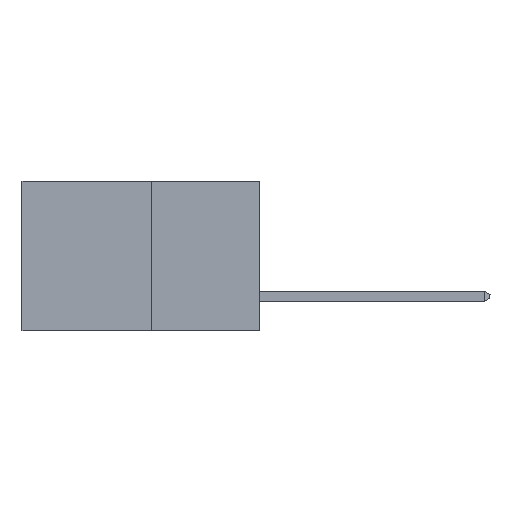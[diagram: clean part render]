
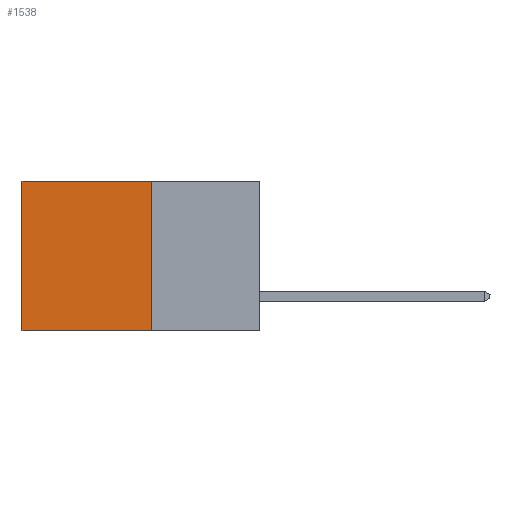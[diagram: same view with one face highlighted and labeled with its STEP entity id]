
A CAD part, left-side view. The second image highlights one B-rep face of the part: STEP entity #1538.
In plain terms, the highlighted planar face has unit normal (-1, 0, 0).
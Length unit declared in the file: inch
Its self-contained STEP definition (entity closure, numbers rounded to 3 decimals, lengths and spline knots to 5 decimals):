
#410 = CARTESIAN_POINT ( 'NONE',  ( 0.277, 0.59, -0.37 ) ) ;
#525 = LINE ( 'NONE', #6794, #6401 ) ;
#628 = CARTESIAN_POINT ( 'NONE',  ( 0.277, 0.27, -0.37 ) ) ;
#763 = CARTESIAN_POINT ( 'NONE',  ( 0.277, 0.27, -0.37 ) ) ;
#1269 = CARTESIAN_POINT ( 'NONE',  ( 0.277, 0.59, 0. ) ) ;
#1388 = DIRECTION ( 'NONE',  ( 1., 0., 0. ) ) ;
#1538 = ADVANCED_FACE ( 'NONE', ( #3960 ), #8419, .F. ) ;
#1837 = VERTEX_POINT ( 'NONE', #410 ) ;
#1838 = DIRECTION ( 'NONE',  ( 0., 1., 0. ) ) ;
#2000 = CARTESIAN_POINT ( 'NONE',  ( 0.277, 0.27, 0. ) ) ;
#2332 = VECTOR ( 'NONE', #1838, 39.37008 ) ;
#2643 = DIRECTION ( 'NONE',  ( 0., 0., -1. ) ) ;
#2728 = EDGE_CURVE ( 'NONE', #9635, #4302, #5594, .T. ) ;
#2854 = EDGE_CURVE ( 'NONE', #9635, #7333, #525, .T. ) ;
#3296 = DIRECTION ( 'NONE',  ( 0., 0., -1. ) ) ;
#3356 = ORIENTED_EDGE ( 'NONE', *, *, #2854, .T. ) ;
#3508 = LINE ( 'NONE', #7505, #7447 ) ;
#3830 = DIRECTION ( 'NONE',  ( 0., 0., -1. ) ) ;
#3960 = FACE_OUTER_BOUND ( 'NONE', #5766, .T. ) ;
#4297 = VECTOR ( 'NONE', #3296, 39.37008 ) ;
#4302 = VERTEX_POINT ( 'NONE', #763 ) ;
#4344 = DIRECTION ( 'NONE',  ( 0., 1., 0. ) ) ;
#4698 = EDGE_CURVE ( 'NONE', #4302, #1837, #6121, .T. ) ;
#5132 = ORIENTED_EDGE ( 'NONE', *, *, #4698, .F. ) ;
#5233 = AXIS2_PLACEMENT_3D ( 'NONE', #628, #1388, #2643 ) ;
#5374 = ORIENTED_EDGE ( 'NONE', *, *, #2728, .F. ) ;
#5594 = LINE ( 'NONE', #8568, #4297 ) ;
#5718 = CARTESIAN_POINT ( 'NONE',  ( 0.277, 0.27, -0.37 ) ) ;
#5766 = EDGE_LOOP ( 'NONE', ( #7102, #5132, #5374, #3356 ) ) ;
#6121 = LINE ( 'NONE', #5718, #2332 ) ;
#6401 = VECTOR ( 'NONE', #4344, 39.37008 ) ;
#6794 = CARTESIAN_POINT ( 'NONE',  ( 0.277, 0.27, 0. ) ) ;
#7102 = ORIENTED_EDGE ( 'NONE', *, *, #9208, .T. ) ;
#7333 = VERTEX_POINT ( 'NONE', #1269 ) ;
#7447 = VECTOR ( 'NONE', #3830, 39.37008 ) ;
#7505 = CARTESIAN_POINT ( 'NONE',  ( 0.277, 0.59, -0.37 ) ) ;
#8419 = PLANE ( 'NONE',  #5233 ) ;
#8568 = CARTESIAN_POINT ( 'NONE',  ( 0.277, 0.27, -0.37 ) ) ;
#9208 = EDGE_CURVE ( 'NONE', #7333, #1837, #3508, .T. ) ;
#9635 = VERTEX_POINT ( 'NONE', #2000 ) ;
